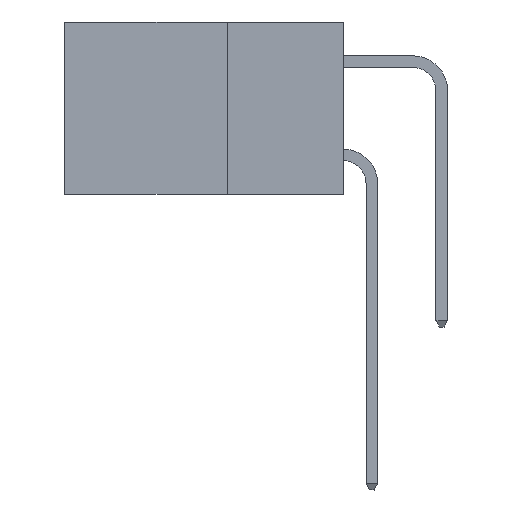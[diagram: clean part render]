
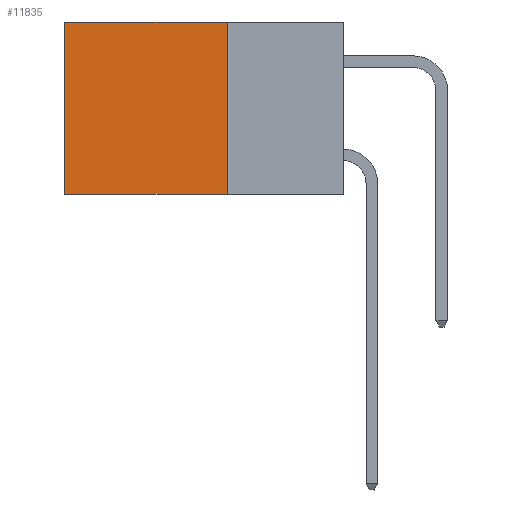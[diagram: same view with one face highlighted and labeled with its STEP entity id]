
A CAD part, left-side view. The second image highlights one B-rep face of the part: STEP entity #11835.
In plain terms, the highlighted planar face has unit normal (-1, 0, 0).
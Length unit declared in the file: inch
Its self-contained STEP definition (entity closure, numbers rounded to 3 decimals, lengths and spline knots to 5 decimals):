
#99 = VECTOR ( 'NONE', #14161, 39.37008 ) ;
#1969 = EDGE_CURVE ( 'NONE', #7959, #10657, #19705, .T. ) ;
#2156 = EDGE_CURVE ( 'NONE', #10496, #10657, #3017, .T. ) ;
#3017 = LINE ( 'NONE', #10958, #99 ) ;
#3663 = DIRECTION ( 'NONE',  ( 1., 0., 0. ) ) ;
#3970 = VECTOR ( 'NONE', #12278, 39.37008 ) ;
#4102 = LINE ( 'NONE', #11967, #6871 ) ;
#4298 = ORIENTED_EDGE ( 'NONE', *, *, #1969, .T. ) ;
#4787 = ORIENTED_EDGE ( 'NONE', *, *, #2156, .F. ) ;
#6730 = VERTEX_POINT ( 'NONE', #11123 ) ;
#6871 = VECTOR ( 'NONE', #12183, 39.37008 ) ;
#7398 = CARTESIAN_POINT ( 'NONE',  ( 0.2615, 0.6, -0.37 ) ) ;
#7774 = CARTESIAN_POINT ( 'NONE',  ( 0.2615, 0.6, 0. ) ) ;
#7959 = VERTEX_POINT ( 'NONE', #7774 ) ;
#9262 = VECTOR ( 'NONE', #13746, 39.37008 ) ;
#9878 = DIRECTION ( 'NONE',  ( 0., 0., -1. ) ) ;
#10425 = LINE ( 'NONE', #19772, #3970 ) ;
#10496 = VERTEX_POINT ( 'NONE', #15805 ) ;
#10657 = VERTEX_POINT ( 'NONE', #15441 ) ;
#10958 = CARTESIAN_POINT ( 'NONE',  ( 0.2615, 0.25, -0.37 ) ) ;
#11123 = CARTESIAN_POINT ( 'NONE',  ( 0.2615, 0.25, 0. ) ) ;
#11835 = ADVANCED_FACE ( 'NONE', ( #12865 ), #15833, .F. ) ;
#11967 = CARTESIAN_POINT ( 'NONE',  ( 0.2615, 0.25, 0. ) ) ;
#12183 = DIRECTION ( 'NONE',  ( 0., 1., 0. ) ) ;
#12278 = DIRECTION ( 'NONE',  ( 0., 0., -1. ) ) ;
#12865 = FACE_OUTER_BOUND ( 'NONE', #19651, .T. ) ;
#13063 = AXIS2_PLACEMENT_3D ( 'NONE', #17469, #3663, #9878 ) ;
#13746 = DIRECTION ( 'NONE',  ( 0., 0., -1. ) ) ;
#14161 = DIRECTION ( 'NONE',  ( 0., 1., 0. ) ) ;
#14438 = EDGE_CURVE ( 'NONE', #6730, #10496, #10425, .T. ) ;
#15441 = CARTESIAN_POINT ( 'NONE',  ( 0.2615, 0.6, -0.37 ) ) ;
#15805 = CARTESIAN_POINT ( 'NONE',  ( 0.2615, 0.25, -0.37 ) ) ;
#15833 = PLANE ( 'NONE',  #13063 ) ;
#16823 = ORIENTED_EDGE ( 'NONE', *, *, #14438, .F. ) ;
#17469 = CARTESIAN_POINT ( 'NONE',  ( 0.2615, 0.25, -0.37 ) ) ;
#17771 = EDGE_CURVE ( 'NONE', #6730, #7959, #4102, .T. ) ;
#19651 = EDGE_LOOP ( 'NONE', ( #4298, #4787, #16823, #20190 ) ) ;
#19705 = LINE ( 'NONE', #7398, #9262 ) ;
#19772 = CARTESIAN_POINT ( 'NONE',  ( 0.2615, 0.25, -0.37 ) ) ;
#20190 = ORIENTED_EDGE ( 'NONE', *, *, #17771, .T. ) ;
